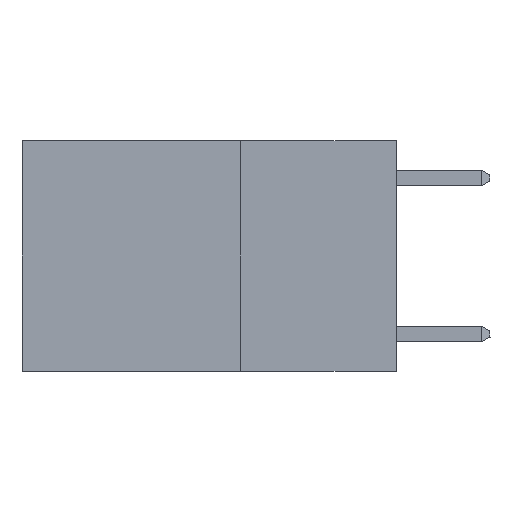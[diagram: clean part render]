
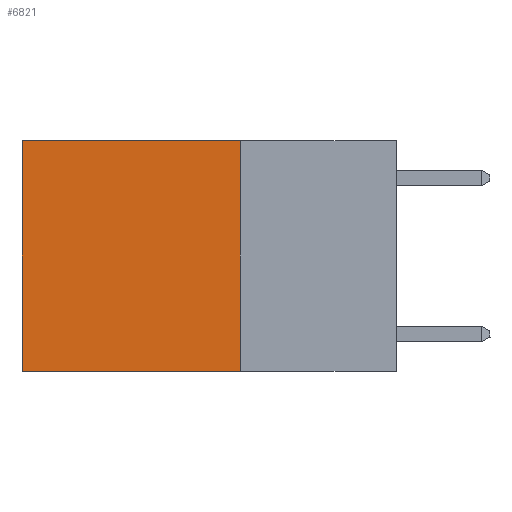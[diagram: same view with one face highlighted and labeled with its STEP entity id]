
A CAD part, left-side view. The second image highlights one B-rep face of the part: STEP entity #6821.
In plain terms, the highlighted planar face has unit normal (-1, 0, 0).
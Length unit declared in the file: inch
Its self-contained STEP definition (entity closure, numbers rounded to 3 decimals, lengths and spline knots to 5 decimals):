
#450 = CARTESIAN_POINT ( 'NONE',  ( 0.2625, 0.25, 0. ) ) ;
#552 = ORIENTED_EDGE ( 'NONE', *, *, #11800, .T. ) ;
#1737 = ORIENTED_EDGE ( 'NONE', *, *, #3457, .F. ) ;
#1843 = LINE ( 'NONE', #7027, #8616 ) ;
#1949 = LINE ( 'NONE', #10193, #9624 ) ;
#2322 = LINE ( 'NONE', #9235, #7679 ) ;
#2819 = AXIS2_PLACEMENT_3D ( 'NONE', #3901, #5980, #12586 ) ;
#3055 = ORIENTED_EDGE ( 'NONE', *, *, #6744, .T. ) ;
#3081 = CARTESIAN_POINT ( 'NONE',  ( 0.2625, 0.25, -0.37 ) ) ;
#3235 = DIRECTION ( 'NONE',  ( 0., 0., -1. ) ) ;
#3246 = DIRECTION ( 'NONE',  ( 0., 1., 0. ) ) ;
#3457 = EDGE_CURVE ( 'NONE', #11009, #7021, #2322, .T. ) ;
#3901 = CARTESIAN_POINT ( 'NONE',  ( 0.2625, 0.25, 0. ) ) ;
#4490 = EDGE_CURVE ( 'NONE', #7021, #12735, #1949, .T. ) ;
#5228 = CARTESIAN_POINT ( 'NONE',  ( 0.2625, 0.6, 0. ) ) ;
#5891 = VECTOR ( 'NONE', #7637, 39.37008 ) ;
#5980 = DIRECTION ( 'NONE',  ( 1., 0., 0. ) ) ;
#6744 = EDGE_CURVE ( 'NONE', #11009, #7665, #7263, .T. ) ;
#6821 = ADVANCED_FACE ( 'NONE', ( #8956 ), #7893, .F. ) ;
#7021 = VERTEX_POINT ( 'NONE', #3081 ) ;
#7027 = CARTESIAN_POINT ( 'NONE',  ( 0.2625, 0.6, 0. ) ) ;
#7128 = CARTESIAN_POINT ( 'NONE',  ( 0.2625, 0.6, -0.37 ) ) ;
#7263 = LINE ( 'NONE', #450, #5891 ) ;
#7637 = DIRECTION ( 'NONE',  ( 0., 1., 0. ) ) ;
#7665 = VERTEX_POINT ( 'NONE', #5228 ) ;
#7679 = VECTOR ( 'NONE', #3235, 39.37008 ) ;
#7893 = PLANE ( 'NONE',  #2819 ) ;
#7923 = CARTESIAN_POINT ( 'NONE',  ( 0.2625, 0.25, 0. ) ) ;
#8616 = VECTOR ( 'NONE', #10822, 39.37008 ) ;
#8956 = FACE_OUTER_BOUND ( 'NONE', #9636, .T. ) ;
#8989 = ORIENTED_EDGE ( 'NONE', *, *, #4490, .F. ) ;
#9235 = CARTESIAN_POINT ( 'NONE',  ( 0.2625, 0.25, 0. ) ) ;
#9624 = VECTOR ( 'NONE', #3246, 39.37008 ) ;
#9636 = EDGE_LOOP ( 'NONE', ( #552, #8989, #1737, #3055 ) ) ;
#10193 = CARTESIAN_POINT ( 'NONE',  ( 0.2625, 0.25, -0.37 ) ) ;
#10822 = DIRECTION ( 'NONE',  ( 0., 0., -1. ) ) ;
#11009 = VERTEX_POINT ( 'NONE', #7923 ) ;
#11800 = EDGE_CURVE ( 'NONE', #7665, #12735, #1843, .T. ) ;
#12586 = DIRECTION ( 'NONE',  ( 0., 0., -1. ) ) ;
#12735 = VERTEX_POINT ( 'NONE', #7128 ) ;
